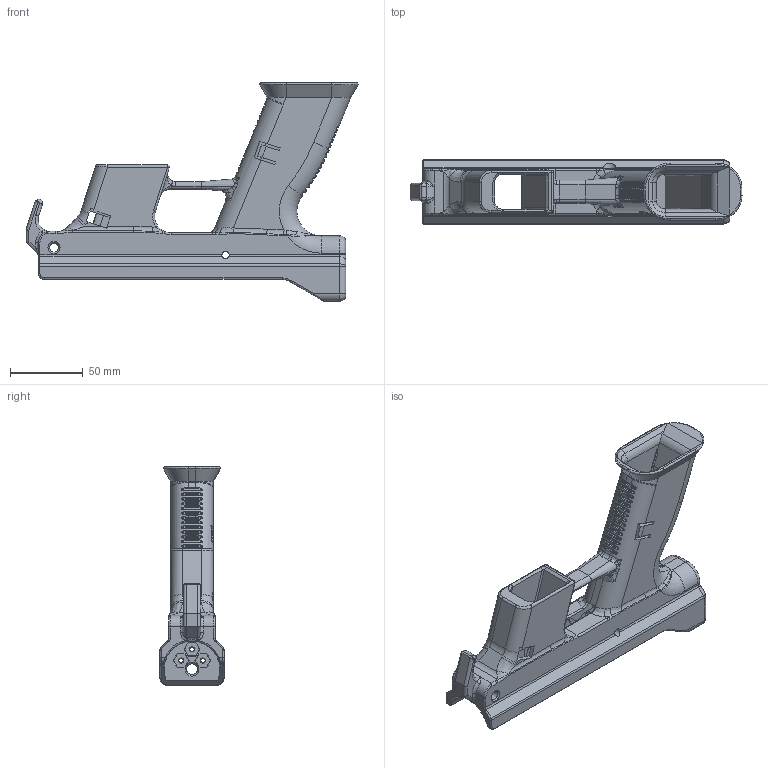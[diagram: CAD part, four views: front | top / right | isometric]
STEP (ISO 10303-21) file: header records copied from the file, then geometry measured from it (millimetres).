
FILE_DESCRIPTION(/* description */ (''),/* implementation_level */ '2;1');
FILE_NAME(/* name */ 'KAP-9 Frame.step',/* time_stamp */ '2021-07-29T03:03:35-04:00',/* author */ (''),/* organization */ (''),/* preprocessor_version */ 'ST-DEVELOPER v18.1',/* originating_system */ 'Autodesk Translation Framework v10.9.0.1377',/* authorisation */ '');
FILE_SCHEMA (('AUTOMOTIVE_DESIGN { 1 0 10303 214 3 1 1 }'));
Products named in the file (2): KAP-9; KAP-9 Frame
Assembly tree (1 placements, depth 2):
  KAP-9
    KAP-9 Frame
Bounding box: 227.94 x 44 x 149.96 mm (x, y, z)
Volume: 240470.4 mm3; surface area: 85278 mm2
Topology: 1 solids, 1 shells, 963 faces, 2603 edges, 1605 vertices
Faces by surface type: bspline 339, plane 288, cylinder 256, torus 58, cone 16, sphere 6
Full cylindrical faces by diameter (mm): 3 x3, 5 x2, 6.3 x2, 7.5 x1
Entity records: 49385 total; most frequent: CARTESIAN_POINT 27066, ORIENTED_EDGE 5154, DIRECTION 4020, EDGE_CURVE 2577, VERTEX_POINT 1605, AXIS2_PLACEMENT_3D 1539, EDGE_LOOP 980, FACE_OUTER_BOUND 963
